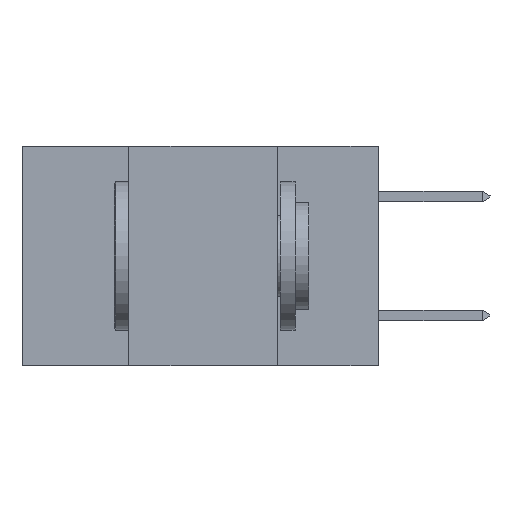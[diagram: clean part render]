
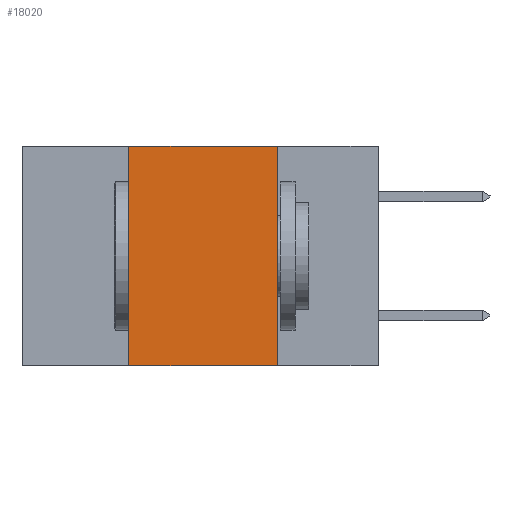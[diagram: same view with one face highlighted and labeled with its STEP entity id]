
A CAD part, left-side view. The second image highlights one B-rep face of the part: STEP entity #18020.
In plain terms, the highlighted planar face has unit normal (-1, 0, 0).
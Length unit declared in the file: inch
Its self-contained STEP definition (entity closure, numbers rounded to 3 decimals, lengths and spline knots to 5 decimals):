
#604 = LINE ( 'NONE', #12229, #16665 ) ;
#1662 = CARTESIAN_POINT ( 'NONE',  ( 0., 0.42, 0. ) ) ;
#1668 = ORIENTED_EDGE ( 'NONE', *, *, #16599, .F. ) ;
#1833 = VECTOR ( 'NONE', #15372, 39.37008 ) ;
#1904 = EDGE_CURVE ( 'NONE', #6490, #7779, #15586, .T. ) ;
#1920 = EDGE_CURVE ( 'NONE', #11380, #15181, #604, .T. ) ;
#2366 = PLANE ( 'NONE',  #14030 ) ;
#2578 = DIRECTION ( 'NONE',  ( 1., 0., 0. ) ) ;
#3914 = DIRECTION ( 'NONE',  ( 0., -1., 0. ) ) ;
#3974 = ORIENTED_EDGE ( 'NONE', *, *, #1920, .T. ) ;
#4076 = DIRECTION ( 'NONE',  ( 0., 0., -1. ) ) ;
#5711 = VECTOR ( 'NONE', #19941, 39.37008 ) ;
#5759 = CARTESIAN_POINT ( 'NONE',  ( 0., 0.42, -0.37 ) ) ;
#6490 = VERTEX_POINT ( 'NONE', #1662 ) ;
#7779 = VERTEX_POINT ( 'NONE', #12509 ) ;
#8390 = LINE ( 'NONE', #13366, #5711 ) ;
#9085 = CARTESIAN_POINT ( 'NONE',  ( 0., 0.6, 0. ) ) ;
#9522 = CARTESIAN_POINT ( 'NONE',  ( 0., 0.42, -0.37 ) ) ;
#10771 = FACE_OUTER_BOUND ( 'NONE', #16824, .T. ) ;
#10822 = DIRECTION ( 'NONE',  ( 0., 0., 1. ) ) ;
#10880 = CARTESIAN_POINT ( 'NONE',  ( 0., 0.17, -0.37 ) ) ;
#11380 = VERTEX_POINT ( 'NONE', #5759 ) ;
#12229 = CARTESIAN_POINT ( 'NONE',  ( 0., 0.6, -0.37 ) ) ;
#12509 = CARTESIAN_POINT ( 'NONE',  ( 0., 0.17, 0. ) ) ;
#13366 = CARTESIAN_POINT ( 'NONE',  ( 0., 0.17, -0.37 ) ) ;
#14030 = AXIS2_PLACEMENT_3D ( 'NONE', #15647, #2578, #4076 ) ;
#14411 = VECTOR ( 'NONE', #10822, 39.37008 ) ;
#15181 = VERTEX_POINT ( 'NONE', #10880 ) ;
#15372 = DIRECTION ( 'NONE',  ( 0., -1., 0. ) ) ;
#15586 = LINE ( 'NONE', #9085, #1833 ) ;
#15647 = CARTESIAN_POINT ( 'NONE',  ( 0., 0.6, 0. ) ) ;
#16599 = EDGE_CURVE ( 'NONE', #7779, #15181, #8390, .T. ) ;
#16665 = VECTOR ( 'NONE', #3914, 39.37008 ) ;
#16824 = EDGE_LOOP ( 'NONE', ( #1668, #20208, #18512, #3974 ) ) ;
#18020 = ADVANCED_FACE ( 'NONE', ( #10771 ), #2366, .F. ) ;
#18512 = ORIENTED_EDGE ( 'NONE', *, *, #20496, .F. ) ;
#19040 = LINE ( 'NONE', #9522, #14411 ) ;
#19941 = DIRECTION ( 'NONE',  ( 0., 0., -1. ) ) ;
#20208 = ORIENTED_EDGE ( 'NONE', *, *, #1904, .F. ) ;
#20496 = EDGE_CURVE ( 'NONE', #11380, #6490, #19040, .T. ) ;
